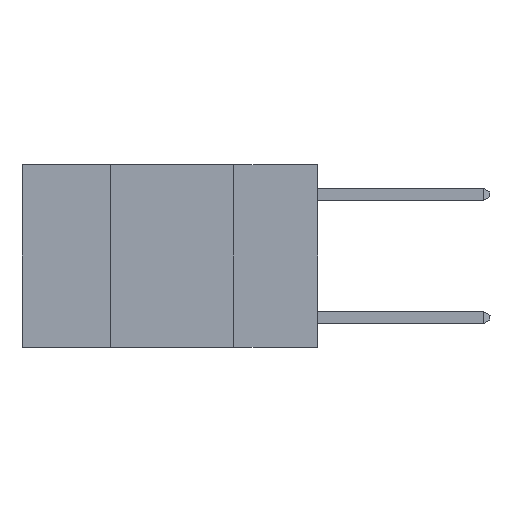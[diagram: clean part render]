
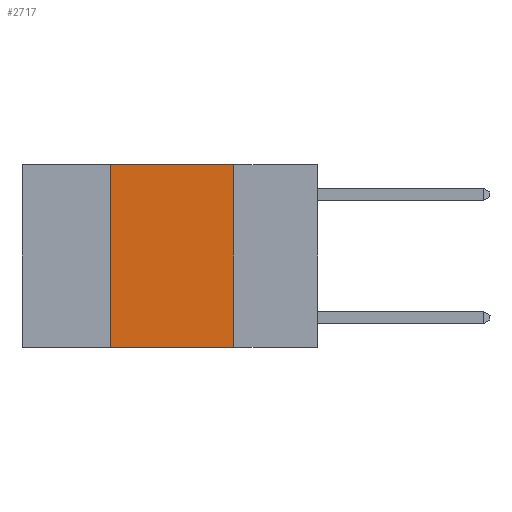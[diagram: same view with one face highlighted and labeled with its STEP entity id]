
A CAD part, left-side view. The second image highlights one B-rep face of the part: STEP entity #2717.
In plain terms, the highlighted planar face has unit normal (-1, 0, 0).
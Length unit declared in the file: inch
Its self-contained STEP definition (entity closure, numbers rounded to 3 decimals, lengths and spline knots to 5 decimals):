
#198 = EDGE_LOOP ( 'NONE', ( #4197, #18065, #24961, #5777 ) ) ;
#483 = EDGE_CURVE ( 'NONE', #11326, #16393, #20289, .T. ) ;
#2539 = VECTOR ( 'NONE', #17397, 39.37008 ) ;
#2650 = CARTESIAN_POINT ( 'NONE',  ( 0., 0.17, 0. ) ) ;
#2717 = ADVANCED_FACE ( 'NONE', ( #4897 ), #14228, .F. ) ;
#3454 = CARTESIAN_POINT ( 'NONE',  ( 0., 0.17, -0.37 ) ) ;
#4113 = DIRECTION ( 'NONE',  ( 0., -1., 0. ) ) ;
#4197 = ORIENTED_EDGE ( 'NONE', *, *, #26582, .F. ) ;
#4897 = FACE_OUTER_BOUND ( 'NONE', #198, .T. ) ;
#5777 = ORIENTED_EDGE ( 'NONE', *, *, #483, .T. ) ;
#7358 = AXIS2_PLACEMENT_3D ( 'NONE', #25905, #30565, #16592 ) ;
#9080 = CARTESIAN_POINT ( 'NONE',  ( 0., 0.42, 0. ) ) ;
#11326 = VERTEX_POINT ( 'NONE', #29653 ) ;
#11395 = LINE ( 'NONE', #27418, #23168 ) ;
#14228 = PLANE ( 'NONE',  #7358 ) ;
#15033 = CARTESIAN_POINT ( 'NONE',  ( 0., 0.42, 0. ) ) ;
#15670 = CARTESIAN_POINT ( 'NONE',  ( 0., 0.6, -0.37 ) ) ;
#16393 = VERTEX_POINT ( 'NONE', #3454 ) ;
#16592 = DIRECTION ( 'NONE',  ( 0., 0., -1. ) ) ;
#17397 = DIRECTION ( 'NONE',  ( 0., 0., 1. ) ) ;
#17410 = LINE ( 'NONE', #25350, #22196 ) ;
#18065 = ORIENTED_EDGE ( 'NONE', *, *, #24634, .F. ) ;
#20289 = LINE ( 'NONE', #15670, #26506 ) ;
#20397 = DIRECTION ( 'NONE',  ( 0., -1., 0. ) ) ;
#21537 = LINE ( 'NONE', #15033, #2539 ) ;
#22196 = VECTOR ( 'NONE', #4113, 39.37008 ) ;
#22732 = DIRECTION ( 'NONE',  ( 0., 0., -1. ) ) ;
#23168 = VECTOR ( 'NONE', #22732, 39.37008 ) ;
#24634 = EDGE_CURVE ( 'NONE', #25365, #28175, #17410, .T. ) ;
#24961 = ORIENTED_EDGE ( 'NONE', *, *, #29697, .F. ) ;
#25350 = CARTESIAN_POINT ( 'NONE',  ( 0., 0.6, 0. ) ) ;
#25365 = VERTEX_POINT ( 'NONE', #9080 ) ;
#25905 = CARTESIAN_POINT ( 'NONE',  ( 0., 0.6, 0. ) ) ;
#26506 = VECTOR ( 'NONE', #20397, 39.37008 ) ;
#26582 = EDGE_CURVE ( 'NONE', #28175, #16393, #11395, .T. ) ;
#27418 = CARTESIAN_POINT ( 'NONE',  ( 0., 0.17, 0. ) ) ;
#28175 = VERTEX_POINT ( 'NONE', #2650 ) ;
#29653 = CARTESIAN_POINT ( 'NONE',  ( 0., 0.42, -0.37 ) ) ;
#29697 = EDGE_CURVE ( 'NONE', #11326, #25365, #21537, .T. ) ;
#30565 = DIRECTION ( 'NONE',  ( 1., 0., 0. ) ) ;
